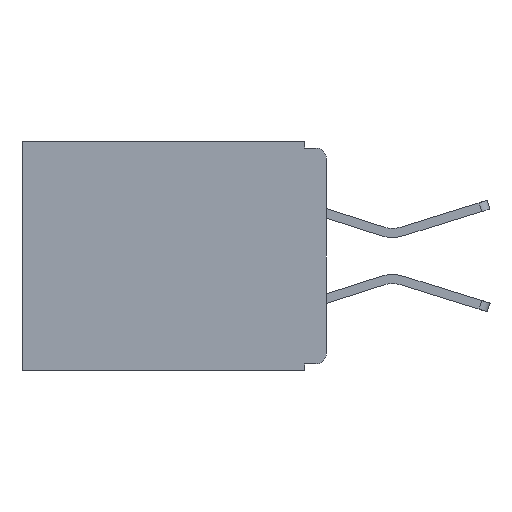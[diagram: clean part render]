
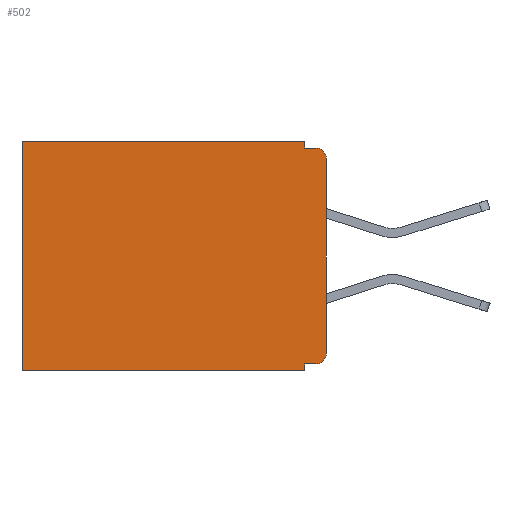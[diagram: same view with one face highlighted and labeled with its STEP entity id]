
A CAD part, left-side view. The second image highlights one B-rep face of the part: STEP entity #502.
In plain terms, the highlighted planar face has unit normal (-1, 0, 0).
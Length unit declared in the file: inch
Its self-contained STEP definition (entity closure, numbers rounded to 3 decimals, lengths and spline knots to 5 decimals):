
#251 = DIRECTION ( 'NONE',  ( 0., 0., -1. ) ) ;
#478 = FACE_OUTER_BOUND ( 'NONE', #3167, .T. ) ;
#502 = ADVANCED_FACE ( 'NONE', ( #478 ), #8989, .F. ) ;
#898 = AXIS2_PLACEMENT_3D ( 'NONE', #9087, #30909, #251 ) ;
#1512 = EDGE_CURVE ( 'NONE', #28730, #4665, #22465, .T. ) ;
#2493 = AXIS2_PLACEMENT_3D ( 'NONE', #17394, #17361, #17329 ) ;
#2913 = CARTESIAN_POINT ( 'NONE',  ( 0.3, 0.015, -0.01 ) ) ;
#3167 = EDGE_LOOP ( 'NONE', ( #33047, #20721, #28025, #20870, #11328, #6148, #12350, #6142, #24853, #29593 ) ) ;
#3879 = VERTEX_POINT ( 'NONE', #28447 ) ;
#3986 = EDGE_CURVE ( 'NONE', #25105, #11075, #31474, .T. ) ;
#4353 = CARTESIAN_POINT ( 'NONE',  ( 0.3, 0., -0.305 ) ) ;
#4602 = CIRCLE ( 'NONE', #2493, 0.015 ) ;
#4665 = VERTEX_POINT ( 'NONE', #19162 ) ;
#4732 = DIRECTION ( 'NONE',  ( 0., 1., 0. ) ) ;
#5092 = VERTEX_POINT ( 'NONE', #20205 ) ;
#5171 = EDGE_CURVE ( 'NONE', #11075, #5092, #21881, .T. ) ;
#6142 = ORIENTED_EDGE ( 'NONE', *, *, #5171, .F. ) ;
#6148 = ORIENTED_EDGE ( 'NONE', *, *, #1512, .T. ) ;
#6224 = CARTESIAN_POINT ( 'NONE',  ( 0.3, 0.031, -0.01 ) ) ;
#6396 = LINE ( 'NONE', #8913, #31363 ) ;
#6436 = CARTESIAN_POINT ( 'NONE',  ( 0.3, 0.015, -0.32 ) ) ;
#6438 = DIRECTION ( 'NONE',  ( 0., -1., 0. ) ) ;
#7776 = VECTOR ( 'NONE', #4732, 39.37008 ) ;
#8032 = CARTESIAN_POINT ( 'NONE',  ( 0.3, 0.031, 0. ) ) ;
#8293 = EDGE_CURVE ( 'NONE', #3879, #12394, #4602, .T. ) ;
#8803 = DIRECTION ( 'NONE',  ( -1., 0., 0. ) ) ;
#8832 = VERTEX_POINT ( 'NONE', #6224 ) ;
#8913 = CARTESIAN_POINT ( 'NONE',  ( 0.3, 0., -0.33 ) ) ;
#8989 = PLANE ( 'NONE',  #898 ) ;
#9087 = CARTESIAN_POINT ( 'NONE',  ( 0.3, 0., -0.33 ) ) ;
#10224 = DIRECTION ( 'NONE',  ( 0., 0., -1. ) ) ;
#10633 = CARTESIAN_POINT ( 'NONE',  ( 0.3, 0.031, -0.33 ) ) ;
#10803 = AXIS2_PLACEMENT_3D ( 'NONE', #24287, #8803, #26854 ) ;
#11075 = VERTEX_POINT ( 'NONE', #15625 ) ;
#11328 = ORIENTED_EDGE ( 'NONE', *, *, #21654, .T. ) ;
#11824 = CARTESIAN_POINT ( 'NONE',  ( 0.3, 0.437, -0.33 ) ) ;
#11950 = VECTOR ( 'NONE', #33267, 39.37008 ) ;
#12350 = ORIENTED_EDGE ( 'NONE', *, *, #14817, .F. ) ;
#12394 = VERTEX_POINT ( 'NONE', #2913 ) ;
#12552 = CARTESIAN_POINT ( 'NONE',  ( 0.3, 0., 0. ) ) ;
#14817 = EDGE_CURVE ( 'NONE', #5092, #4665, #6396, .T. ) ;
#15302 = VECTOR ( 'NONE', #10224, 39.37008 ) ;
#15615 = VECTOR ( 'NONE', #22369, 39.37008 ) ;
#15625 = CARTESIAN_POINT ( 'NONE',  ( 0.3, 0.031, -0.32 ) ) ;
#15820 = VECTOR ( 'NONE', #32129, 39.37008 ) ;
#16118 = LINE ( 'NONE', #25813, #15302 ) ;
#16408 = VERTEX_POINT ( 'NONE', #8032 ) ;
#17329 = DIRECTION ( 'NONE',  ( 0., 0., -1. ) ) ;
#17361 = DIRECTION ( 'NONE',  ( -1., 0., 0. ) ) ;
#17394 = CARTESIAN_POINT ( 'NONE',  ( 0.3, 0.015, -0.025 ) ) ;
#17423 = EDGE_CURVE ( 'NONE', #3879, #32762, #32384, .T. ) ;
#17895 = DIRECTION ( 'NONE',  ( 0., 1., 0. ) ) ;
#19162 = CARTESIAN_POINT ( 'NONE',  ( 0.3, 0.437, -0.33 ) ) ;
#19563 = EDGE_CURVE ( 'NONE', #8832, #12394, #31254, .T. ) ;
#20205 = CARTESIAN_POINT ( 'NONE',  ( 0.3, 0.031, -0.33 ) ) ;
#20721 = ORIENTED_EDGE ( 'NONE', *, *, #8293, .T. ) ;
#20870 = ORIENTED_EDGE ( 'NONE', *, *, #24289, .F. ) ;
#21608 = LINE ( 'NONE', #12552, #7776 ) ;
#21654 = EDGE_CURVE ( 'NONE', #16408, #28730, #21608, .T. ) ;
#21796 = CARTESIAN_POINT ( 'NONE',  ( 0.3, 0., -0.01 ) ) ;
#21881 = LINE ( 'NONE', #10633, #15820 ) ;
#22369 = DIRECTION ( 'NONE',  ( 0., 0., -1. ) ) ;
#22465 = LINE ( 'NONE', #11824, #15615 ) ;
#24287 = CARTESIAN_POINT ( 'NONE',  ( 0.3, 0.015, -0.305 ) ) ;
#24289 = EDGE_CURVE ( 'NONE', #16408, #8832, #16118, .T. ) ;
#24515 = VECTOR ( 'NONE', #6438, 39.37008 ) ;
#24734 = VECTOR ( 'NONE', #17895, 39.37008 ) ;
#24853 = ORIENTED_EDGE ( 'NONE', *, *, #3986, .F. ) ;
#25105 = VERTEX_POINT ( 'NONE', #6436 ) ;
#25701 = EDGE_CURVE ( 'NONE', #25105, #32762, #27080, .T. ) ;
#25813 = CARTESIAN_POINT ( 'NONE',  ( 0.3, 0.031, 0. ) ) ;
#26031 = CARTESIAN_POINT ( 'NONE',  ( 0.3, 0.437, 0. ) ) ;
#26854 = DIRECTION ( 'NONE',  ( 0., 0., -1. ) ) ;
#26962 = DIRECTION ( 'NONE',  ( 0., 1., 0. ) ) ;
#27080 = CIRCLE ( 'NONE', #10803, 0.015 ) ;
#28025 = ORIENTED_EDGE ( 'NONE', *, *, #19563, .F. ) ;
#28239 = CARTESIAN_POINT ( 'NONE',  ( 0.3, 0., -0.33 ) ) ;
#28447 = CARTESIAN_POINT ( 'NONE',  ( 0.3, 0., -0.025 ) ) ;
#28730 = VERTEX_POINT ( 'NONE', #26031 ) ;
#28944 = CARTESIAN_POINT ( 'NONE',  ( 0.3, 0., -0.32 ) ) ;
#29593 = ORIENTED_EDGE ( 'NONE', *, *, #25701, .T. ) ;
#30909 = DIRECTION ( 'NONE',  ( 1., 0., 0. ) ) ;
#31254 = LINE ( 'NONE', #21796, #24515 ) ;
#31363 = VECTOR ( 'NONE', #26962, 39.37008 ) ;
#31474 = LINE ( 'NONE', #28944, #24734 ) ;
#32129 = DIRECTION ( 'NONE',  ( 0., 0., -1. ) ) ;
#32384 = LINE ( 'NONE', #28239, #11950 ) ;
#32762 = VERTEX_POINT ( 'NONE', #4353 ) ;
#33047 = ORIENTED_EDGE ( 'NONE', *, *, #17423, .F. ) ;
#33267 = DIRECTION ( 'NONE',  ( 0., 0., -1. ) ) ;
